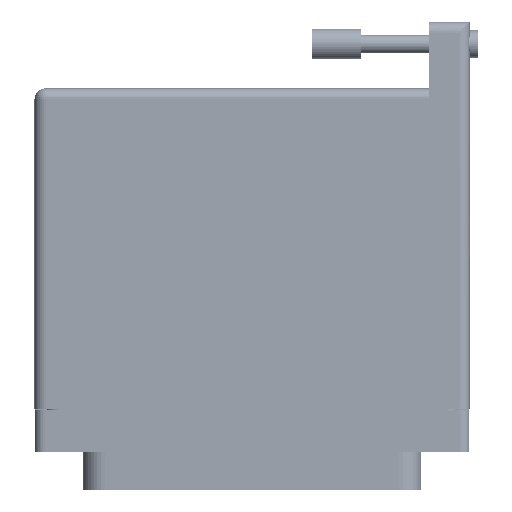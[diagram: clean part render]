
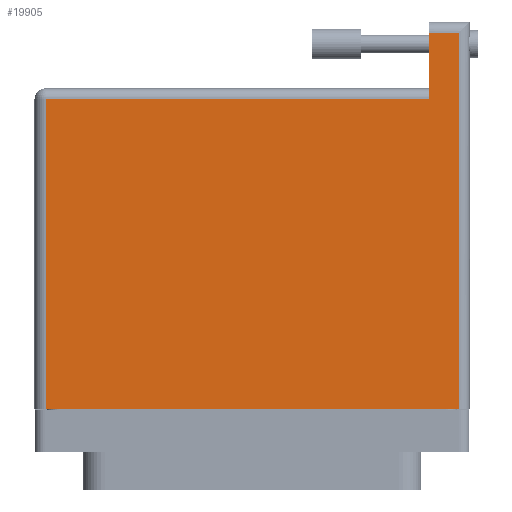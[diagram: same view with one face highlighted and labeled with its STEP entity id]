
A CAD part, front view. The second image highlights one B-rep face of the part: STEP entity #19905.
In plain terms, the highlighted face is planar.
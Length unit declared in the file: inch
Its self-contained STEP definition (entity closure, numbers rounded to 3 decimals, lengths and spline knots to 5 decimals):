
#607 = CARTESIAN_POINT ( 'NONE',  ( -1.3775, 1.86, 0.765 ) ) ;
#3815 = LINE ( 'NONE', #33960, #46333 ) ;
#4386 = DIRECTION ( 'NONE',  ( 0., -1., 0. ) ) ;
#8353 = LINE ( 'NONE', #607, #12829 ) ;
#9427 = VECTOR ( 'NONE', #92438, 39.37008 ) ;
#9914 = AXIS2_PLACEMENT_3D ( 'NONE', #58448, #14684, #79126 ) ;
#12829 = VECTOR ( 'NONE', #64417, 39.37008 ) ;
#13141 = VECTOR ( 'NONE', #48469, 39.37008 ) ;
#14684 = DIRECTION ( 'NONE',  ( 0., 0., -1. ) ) ;
#14912 = CARTESIAN_POINT ( 'NONE',  ( -1.3075, -0.1, 0.765 ) ) ;
#15543 = EDGE_LOOP ( 'NONE', ( #17224, #32674, #36612, #56232, #21915, #69033 ) ) ;
#15750 = CARTESIAN_POINT ( 'NONE',  ( 1.3075, -0.1, 0.765 ) ) ;
#17224 = ORIENTED_EDGE ( 'NONE', *, *, #65962, .T. ) ;
#18225 = CARTESIAN_POINT ( 'NONE',  ( -1.3775, -0.1, 0.765 ) ) ;
#19905 = ADVANCED_FACE ( 'NONE', ( #54913 ), #22170, .F. ) ;
#21915 = ORIENTED_EDGE ( 'NONE', *, *, #36712, .T. ) ;
#22170 = PLANE ( 'NONE',  #9914 ) ;
#23726 = VERTEX_POINT ( 'NONE', #52787 ) ;
#24975 = CARTESIAN_POINT ( 'NONE',  ( 1.1215, 2.28, 0.765 ) ) ;
#26395 = DIRECTION ( 'NONE',  ( 0., 1., 0. ) ) ;
#27397 = CARTESIAN_POINT ( 'NONE',  ( -1.3075, -0.1, 0.765 ) ) ;
#32140 = EDGE_CURVE ( 'NONE', #85558, #64425, #88809, .T. ) ;
#32191 = LINE ( 'NONE', #56280, #13141 ) ;
#32646 = DIRECTION ( 'NONE',  ( 1., 0., 0. ) ) ;
#32674 = ORIENTED_EDGE ( 'NONE', *, *, #84154, .T. ) ;
#33960 = CARTESIAN_POINT ( 'NONE',  ( 1.3075, 2.35, 0.765 ) ) ;
#36612 = ORIENTED_EDGE ( 'NONE', *, *, #32140, .T. ) ;
#36712 = EDGE_CURVE ( 'NONE', #81790, #80139, #3815, .T. ) ;
#39364 = CARTESIAN_POINT ( 'NONE',  ( 1.3075, 2.28, 0.765 ) ) ;
#42780 = VECTOR ( 'NONE', #32646, 39.37008 ) ;
#45305 = CARTESIAN_POINT ( 'NONE',  ( -1.3075, 1.86, 0.765 ) ) ;
#46333 = VECTOR ( 'NONE', #26395, 39.37008 ) ;
#48469 = DIRECTION ( 'NONE',  ( -1., 0., 0. ) ) ;
#52787 = CARTESIAN_POINT ( 'NONE',  ( 1.1215, 1.86, 0.765 ) ) ;
#53356 = EDGE_CURVE ( 'NONE', #64425, #81790, #90835, .T. ) ;
#54913 = FACE_OUTER_BOUND ( 'NONE', #15543, .T. ) ;
#55009 = LINE ( 'NONE', #82857, #59521 ) ;
#56232 = ORIENTED_EDGE ( 'NONE', *, *, #53356, .T. ) ;
#56280 = CARTESIAN_POINT ( 'NONE',  ( -1.3775, 2.28, 0.765 ) ) ;
#58448 = CARTESIAN_POINT ( 'NONE',  ( -1.3775, 1.93, 0.765 ) ) ;
#59521 = VECTOR ( 'NONE', #4386, 39.37008 ) ;
#64417 = DIRECTION ( 'NONE',  ( -1., 0., 0. ) ) ;
#64425 = VERTEX_POINT ( 'NONE', #14912 ) ;
#65962 = EDGE_CURVE ( 'NONE', #84268, #23726, #55009, .T. ) ;
#69033 = ORIENTED_EDGE ( 'NONE', *, *, #73847, .T. ) ;
#73847 = EDGE_CURVE ( 'NONE', #80139, #84268, #32191, .T. ) ;
#79126 = DIRECTION ( 'NONE',  ( -1., 0., 0. ) ) ;
#80139 = VERTEX_POINT ( 'NONE', #39364 ) ;
#81790 = VERTEX_POINT ( 'NONE', #15750 ) ;
#82857 = CARTESIAN_POINT ( 'NONE',  ( 1.1215, 2.35, 0.765 ) ) ;
#84154 = EDGE_CURVE ( 'NONE', #23726, #85558, #8353, .T. ) ;
#84268 = VERTEX_POINT ( 'NONE', #24975 ) ;
#85558 = VERTEX_POINT ( 'NONE', #45305 ) ;
#88809 = LINE ( 'NONE', #27397, #9427 ) ;
#90835 = LINE ( 'NONE', #18225, #42780 ) ;
#92438 = DIRECTION ( 'NONE',  ( 0., -1., 0. ) ) ;
